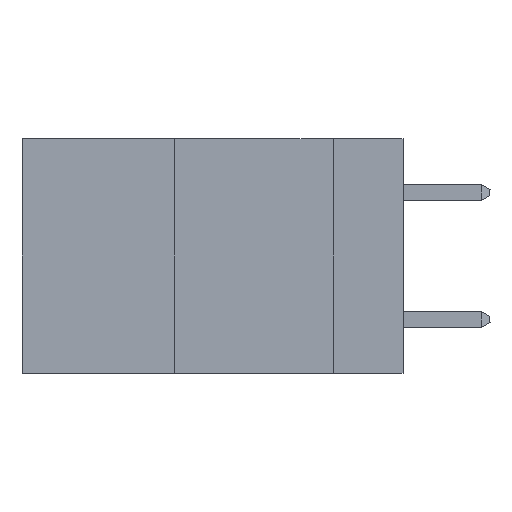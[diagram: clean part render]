
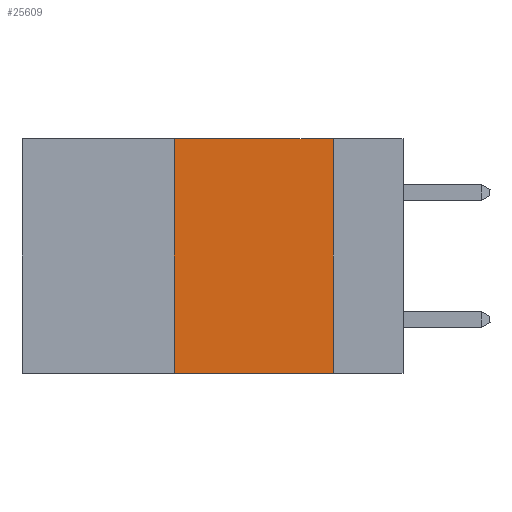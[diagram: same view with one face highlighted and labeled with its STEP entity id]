
A CAD part, left-side view. The second image highlights one B-rep face of the part: STEP entity #25609.
In plain terms, the highlighted planar face has unit normal (-1, 0, 0).
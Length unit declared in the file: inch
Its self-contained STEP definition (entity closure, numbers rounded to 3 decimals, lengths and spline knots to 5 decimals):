
#260 = DIRECTION ( 'NONE',  ( 0., 0., -1. ) ) ;
#4931 = CARTESIAN_POINT ( 'NONE',  ( 0., 0.11, 0. ) ) ;
#4950 = PLANE ( 'NONE',  #33017 ) ;
#5934 = ORIENTED_EDGE ( 'NONE', *, *, #19153, .F. ) ;
#6020 = VERTEX_POINT ( 'NONE', #11049 ) ;
#6879 = EDGE_CURVE ( 'NONE', #6020, #34124, #36339, .T. ) ;
#7878 = DIRECTION ( 'NONE',  ( 0., -1., 0. ) ) ;
#8559 = VECTOR ( 'NONE', #15666, 39.37008 ) ;
#9856 = CARTESIAN_POINT ( 'NONE',  ( 0., 0.36, 0. ) ) ;
#10852 = LINE ( 'NONE', #10897, #39906 ) ;
#10897 = CARTESIAN_POINT ( 'NONE',  ( 0., 0.11, 0. ) ) ;
#11049 = CARTESIAN_POINT ( 'NONE',  ( 0., 0.36, -0.37 ) ) ;
#11517 = CARTESIAN_POINT ( 'NONE',  ( 0., 0.11, -0.37 ) ) ;
#13607 = VECTOR ( 'NONE', #7878, 39.37008 ) ;
#14858 = EDGE_CURVE ( 'NONE', #38624, #34124, #10852, .T. ) ;
#14878 = ORIENTED_EDGE ( 'NONE', *, *, #33649, .F. ) ;
#15278 = DIRECTION ( 'NONE',  ( 0., 0., -1. ) ) ;
#15666 = DIRECTION ( 'NONE',  ( 0., 0., 1. ) ) ;
#18889 = FACE_OUTER_BOUND ( 'NONE', #20586, .T. ) ;
#19153 = EDGE_CURVE ( 'NONE', #37138, #38624, #36063, .T. ) ;
#20250 = ORIENTED_EDGE ( 'NONE', *, *, #14858, .F. ) ;
#20586 = EDGE_LOOP ( 'NONE', ( #20250, #5934, #14878, #42838 ) ) ;
#23878 = LINE ( 'NONE', #9856, #8559 ) ;
#25609 = ADVANCED_FACE ( 'NONE', ( #18889 ), #4950, .F. ) ;
#28363 = CARTESIAN_POINT ( 'NONE',  ( 0., 0.6, -0.37 ) ) ;
#32071 = DIRECTION ( 'NONE',  ( 0., -1., 0. ) ) ;
#32096 = CARTESIAN_POINT ( 'NONE',  ( 0., 0.36, 0. ) ) ;
#32606 = DIRECTION ( 'NONE',  ( 1., 0., 0. ) ) ;
#33017 = AXIS2_PLACEMENT_3D ( 'NONE', #40101, #32606, #15278 ) ;
#33649 = EDGE_CURVE ( 'NONE', #6020, #37138, #23878, .T. ) ;
#34124 = VERTEX_POINT ( 'NONE', #11517 ) ;
#36063 = LINE ( 'NONE', #36070, #13607 ) ;
#36070 = CARTESIAN_POINT ( 'NONE',  ( 0., 0.6, 0. ) ) ;
#36339 = LINE ( 'NONE', #28363, #42397 ) ;
#37138 = VERTEX_POINT ( 'NONE', #32096 ) ;
#38624 = VERTEX_POINT ( 'NONE', #4931 ) ;
#39906 = VECTOR ( 'NONE', #260, 39.37008 ) ;
#40101 = CARTESIAN_POINT ( 'NONE',  ( 0., 0.6, 0. ) ) ;
#42397 = VECTOR ( 'NONE', #32071, 39.37008 ) ;
#42838 = ORIENTED_EDGE ( 'NONE', *, *, #6879, .T. ) ;
